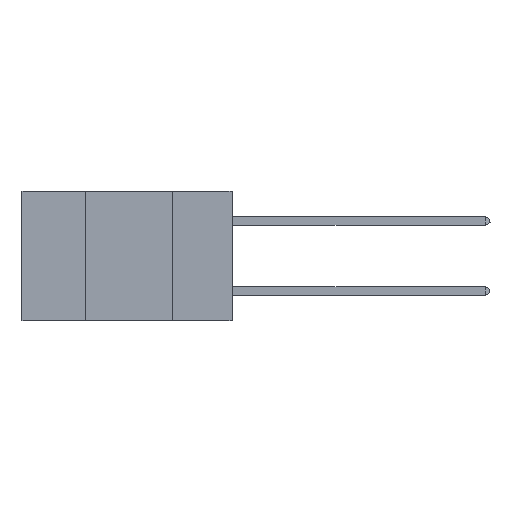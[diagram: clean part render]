
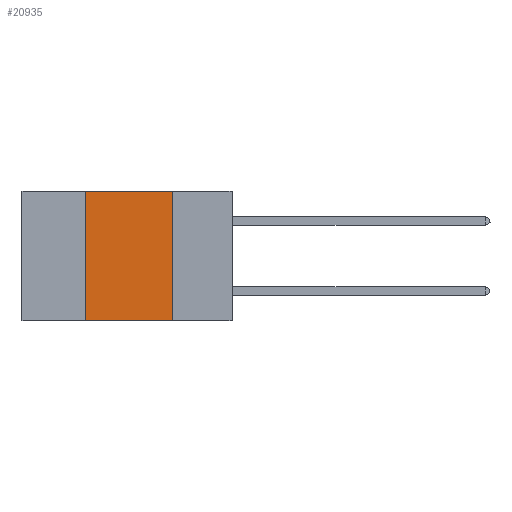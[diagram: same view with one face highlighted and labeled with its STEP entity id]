
A CAD part, left-side view. The second image highlights one B-rep face of the part: STEP entity #20935.
In plain terms, the highlighted planar face has unit normal (-1, 0, 0).
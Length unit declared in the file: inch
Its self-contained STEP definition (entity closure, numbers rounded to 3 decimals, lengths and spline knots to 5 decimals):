
#1278 = CARTESIAN_POINT ( 'NONE',  ( 0., 0.6, 0. ) ) ;
#1894 = EDGE_CURVE ( 'NONE', #17036, #13955, #11456, .T. ) ;
#2380 = CARTESIAN_POINT ( 'NONE',  ( 0., 0.42, 0. ) ) ;
#3304 = DIRECTION ( 'NONE',  ( 0., 0., -1. ) ) ;
#3405 = EDGE_CURVE ( 'NONE', #23973, #17036, #7731, .T. ) ;
#4000 = CARTESIAN_POINT ( 'NONE',  ( 0., 0.17, -0.37 ) ) ;
#4376 = DIRECTION ( 'NONE',  ( 0., 0., 1. ) ) ;
#7731 = LINE ( 'NONE', #2380, #17643 ) ;
#8080 = VECTOR ( 'NONE', #19086, 39.37008 ) ;
#9078 = CARTESIAN_POINT ( 'NONE',  ( 0., 0.6, -0.37 ) ) ;
#9243 = CARTESIAN_POINT ( 'NONE',  ( 0., 0.17, 0. ) ) ;
#9322 = CARTESIAN_POINT ( 'NONE',  ( 0., 0.6, 0. ) ) ;
#10422 = EDGE_LOOP ( 'NONE', ( #12759, #23135, #23727, #13981 ) ) ;
#11019 = VECTOR ( 'NONE', #11100, 39.37008 ) ;
#11100 = DIRECTION ( 'NONE',  ( 0., -1., 0. ) ) ;
#11257 = PLANE ( 'NONE',  #23459 ) ;
#11456 = LINE ( 'NONE', #9322, #16671 ) ;
#12091 = EDGE_CURVE ( 'NONE', #23973, #22980, #21481, .T. ) ;
#12759 = ORIENTED_EDGE ( 'NONE', *, *, #22759, .F. ) ;
#13955 = VERTEX_POINT ( 'NONE', #23721 ) ;
#13981 = ORIENTED_EDGE ( 'NONE', *, *, #12091, .T. ) ;
#14739 = FACE_OUTER_BOUND ( 'NONE', #10422, .T. ) ;
#15242 = DIRECTION ( 'NONE',  ( 1., 0., 0. ) ) ;
#15332 = DIRECTION ( 'NONE',  ( 0., -1., 0. ) ) ;
#16671 = VECTOR ( 'NONE', #15332, 39.37008 ) ;
#17036 = VERTEX_POINT ( 'NONE', #18767 ) ;
#17643 = VECTOR ( 'NONE', #4376, 39.37008 ) ;
#18686 = CARTESIAN_POINT ( 'NONE',  ( 0., 0.42, -0.37 ) ) ;
#18767 = CARTESIAN_POINT ( 'NONE',  ( 0., 0.42, 0. ) ) ;
#19086 = DIRECTION ( 'NONE',  ( 0., 0., -1. ) ) ;
#20935 = ADVANCED_FACE ( 'NONE', ( #14739 ), #11257, .F. ) ;
#21481 = LINE ( 'NONE', #9078, #11019 ) ;
#22759 = EDGE_CURVE ( 'NONE', #13955, #22980, #23759, .T. ) ;
#22980 = VERTEX_POINT ( 'NONE', #4000 ) ;
#23135 = ORIENTED_EDGE ( 'NONE', *, *, #1894, .F. ) ;
#23459 = AXIS2_PLACEMENT_3D ( 'NONE', #1278, #15242, #3304 ) ;
#23721 = CARTESIAN_POINT ( 'NONE',  ( 0., 0.17, 0. ) ) ;
#23727 = ORIENTED_EDGE ( 'NONE', *, *, #3405, .F. ) ;
#23759 = LINE ( 'NONE', #9243, #8080 ) ;
#23973 = VERTEX_POINT ( 'NONE', #18686 ) ;
